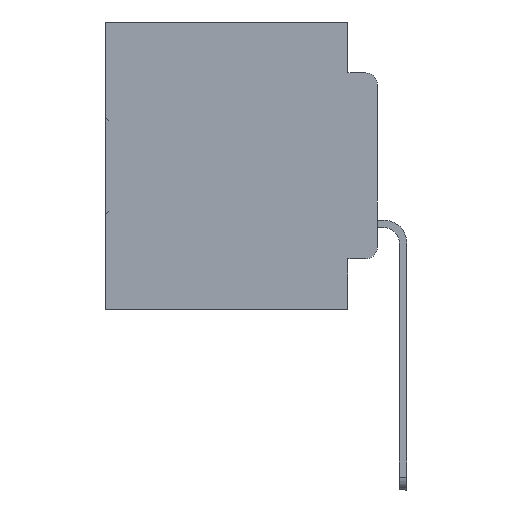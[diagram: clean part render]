
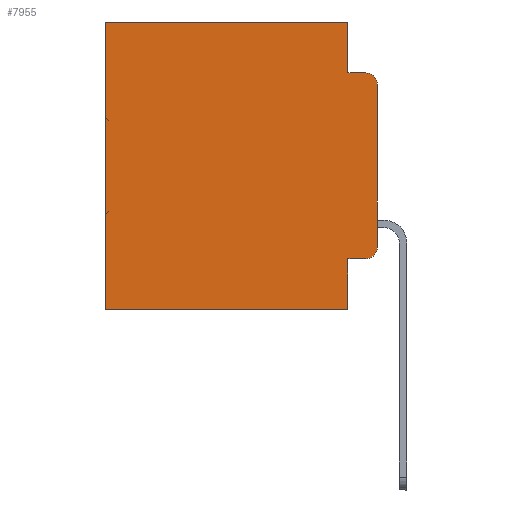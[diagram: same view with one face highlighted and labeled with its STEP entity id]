
A CAD part, left-side view. The second image highlights one B-rep face of the part: STEP entity #7955.
In plain terms, the highlighted planar face has unit normal (-1, 0, 0).
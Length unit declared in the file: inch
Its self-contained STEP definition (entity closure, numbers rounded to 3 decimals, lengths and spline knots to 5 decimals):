
#203 = CARTESIAN_POINT ( 'NONE',  ( 0.298, 0., 0. ) ) ;
#820 = ORIENTED_EDGE ( 'NONE', *, *, #14300, .F. ) ;
#1054 = AXIS2_PLACEMENT_3D ( 'NONE', #17752, #34135, #28851 ) ;
#1495 = EDGE_CURVE ( 'NONE', #8597, #2924, #11210, .T. ) ;
#1567 = CARTESIAN_POINT ( 'NONE',  ( 0.298, 0.051, -0.0885 ) ) ;
#1728 = LINE ( 'NONE', #12062, #14275 ) ;
#2924 = VERTEX_POINT ( 'NONE', #33901 ) ;
#3067 = CARTESIAN_POINT ( 'NONE',  ( 0.298, 0., 0. ) ) ;
#3263 = ORIENTED_EDGE ( 'NONE', *, *, #34142, .T. ) ;
#3347 = CARTESIAN_POINT ( 'NONE',  ( 0.298, 0.051, -0.4115 ) ) ;
#4221 = EDGE_CURVE ( 'NONE', #25596, #11453, #21145, .T. ) ;
#4248 = FACE_OUTER_BOUND ( 'NONE', #35100, .T. ) ;
#4443 = VERTEX_POINT ( 'NONE', #27710 ) ;
#4457 = CARTESIAN_POINT ( 'NONE',  ( 0.298, 0.051, -0.0885 ) ) ;
#5435 = CARTESIAN_POINT ( 'NONE',  ( 0.298, 0.051, -0.5 ) ) ;
#5634 = LINE ( 'NONE', #203, #35762 ) ;
#6344 = VECTOR ( 'NONE', #6651, 39.37008 ) ;
#6446 = DIRECTION ( 'NONE',  ( 0., 0., -1. ) ) ;
#6651 = DIRECTION ( 'NONE',  ( 0., -1., 0. ) ) ;
#7070 = ORIENTED_EDGE ( 'NONE', *, *, #20504, .F. ) ;
#7514 = EDGE_CURVE ( 'NONE', #14577, #27002, #10086, .T. ) ;
#7955 = ADVANCED_FACE ( 'NONE', ( #4248 ), #31304, .F. ) ;
#8597 = VERTEX_POINT ( 'NONE', #25383 ) ;
#9858 = CARTESIAN_POINT ( 'NONE',  ( 0.298, 0.051, 0. ) ) ;
#10086 = LINE ( 'NONE', #23481, #6344 ) ;
#11210 = CIRCLE ( 'NONE', #35542, 0.02 ) ;
#11374 = LINE ( 'NONE', #22423, #25037 ) ;
#11453 = VERTEX_POINT ( 'NONE', #15025 ) ;
#12062 = CARTESIAN_POINT ( 'NONE',  ( 0.298, 0.051, 0. ) ) ;
#13030 = CARTESIAN_POINT ( 'NONE',  ( 0.298, 0.02, -0.1085 ) ) ;
#13315 = AXIS2_PLACEMENT_3D ( 'NONE', #15277, #32005, #6446 ) ;
#13585 = DIRECTION ( 'NONE',  ( 0., 1., 0. ) ) ;
#14071 = CARTESIAN_POINT ( 'NONE',  ( 0.298, 0.02, -0.4115 ) ) ;
#14275 = VECTOR ( 'NONE', #23109, 39.37008 ) ;
#14300 = EDGE_CURVE ( 'NONE', #28600, #2924, #34569, .T. ) ;
#14338 = EDGE_CURVE ( 'NONE', #14577, #25596, #1728, .T. ) ;
#14363 = CIRCLE ( 'NONE', #1054, 0.02 ) ;
#14577 = VERTEX_POINT ( 'NONE', #3347 ) ;
#14741 = DIRECTION ( 'NONE',  ( 0., 0., -1. ) ) ;
#15025 = CARTESIAN_POINT ( 'NONE',  ( 0.298, 0.473, -0.5 ) ) ;
#15277 = CARTESIAN_POINT ( 'NONE',  ( 0.298, 0., 0. ) ) ;
#15993 = ORIENTED_EDGE ( 'NONE', *, *, #4221, .F. ) ;
#17359 = VERTEX_POINT ( 'NONE', #23245 ) ;
#17752 = CARTESIAN_POINT ( 'NONE',  ( 0.298, 0.02, -0.3915 ) ) ;
#18723 = ORIENTED_EDGE ( 'NONE', *, *, #33103, .T. ) ;
#19330 = DIRECTION ( 'NONE',  ( 0., 0., -1. ) ) ;
#19880 = EDGE_CURVE ( 'NONE', #17359, #11453, #11374, .T. ) ;
#20004 = CARTESIAN_POINT ( 'NONE',  ( 0.298, 0., -0.3915 ) ) ;
#20504 = EDGE_CURVE ( 'NONE', #4443, #28600, #28910, .T. ) ;
#20802 = CARTESIAN_POINT ( 'NONE',  ( 0.298, 0., -0.5 ) ) ;
#21145 = LINE ( 'NONE', #20802, #33465 ) ;
#21371 = DIRECTION ( 'NONE',  ( -1., 0., 0. ) ) ;
#21908 = LINE ( 'NONE', #3067, #28206 ) ;
#22423 = CARTESIAN_POINT ( 'NONE',  ( 0.298, 0.473, 0. ) ) ;
#22451 = DIRECTION ( 'NONE',  ( 0., 0., -1. ) ) ;
#23109 = DIRECTION ( 'NONE',  ( 0., 0., -1. ) ) ;
#23245 = CARTESIAN_POINT ( 'NONE',  ( 0.298, 0.473, 0. ) ) ;
#23339 = VERTEX_POINT ( 'NONE', #20004 ) ;
#23481 = CARTESIAN_POINT ( 'NONE',  ( 0.298, 0.051, -0.4115 ) ) ;
#24159 = ORIENTED_EDGE ( 'NONE', *, *, #25599, .F. ) ;
#24451 = DIRECTION ( 'NONE',  ( 0., 0., -1. ) ) ;
#25037 = VECTOR ( 'NONE', #19330, 39.37008 ) ;
#25280 = VECTOR ( 'NONE', #28936, 39.37008 ) ;
#25383 = CARTESIAN_POINT ( 'NONE',  ( 0.298, 0., -0.1085 ) ) ;
#25596 = VERTEX_POINT ( 'NONE', #5435 ) ;
#25599 = EDGE_CURVE ( 'NONE', #8597, #23339, #21908, .T. ) ;
#27002 = VERTEX_POINT ( 'NONE', #14071 ) ;
#27710 = CARTESIAN_POINT ( 'NONE',  ( 0.298, 0.051, 0. ) ) ;
#28206 = VECTOR ( 'NONE', #22451, 39.37008 ) ;
#28600 = VERTEX_POINT ( 'NONE', #1567 ) ;
#28642 = ORIENTED_EDGE ( 'NONE', *, *, #1495, .T. ) ;
#28851 = DIRECTION ( 'NONE',  ( 0., 0., -1. ) ) ;
#28910 = LINE ( 'NONE', #9858, #34353 ) ;
#28936 = DIRECTION ( 'NONE',  ( 0., -1., 0. ) ) ;
#30346 = ORIENTED_EDGE ( 'NONE', *, *, #14338, .F. ) ;
#30849 = ORIENTED_EDGE ( 'NONE', *, *, #19880, .T. ) ;
#31304 = PLANE ( 'NONE',  #13315 ) ;
#32005 = DIRECTION ( 'NONE',  ( 1., 0., 0. ) ) ;
#33103 = EDGE_CURVE ( 'NONE', #4443, #17359, #5634, .T. ) ;
#33216 = ORIENTED_EDGE ( 'NONE', *, *, #7514, .T. ) ;
#33465 = VECTOR ( 'NONE', #34439, 39.37008 ) ;
#33901 = CARTESIAN_POINT ( 'NONE',  ( 0.298, 0.02, -0.0885 ) ) ;
#34135 = DIRECTION ( 'NONE',  ( -1., 0., 0. ) ) ;
#34142 = EDGE_CURVE ( 'NONE', #27002, #23339, #14363, .T. ) ;
#34353 = VECTOR ( 'NONE', #14741, 39.37008 ) ;
#34439 = DIRECTION ( 'NONE',  ( 0., 1., 0. ) ) ;
#34569 = LINE ( 'NONE', #4457, #25280 ) ;
#35100 = EDGE_LOOP ( 'NONE', ( #24159, #28642, #820, #7070, #18723, #30849, #15993, #30346, #33216, #3263 ) ) ;
#35542 = AXIS2_PLACEMENT_3D ( 'NONE', #13030, #21371, #24451 ) ;
#35762 = VECTOR ( 'NONE', #13585, 39.37008 ) ;
